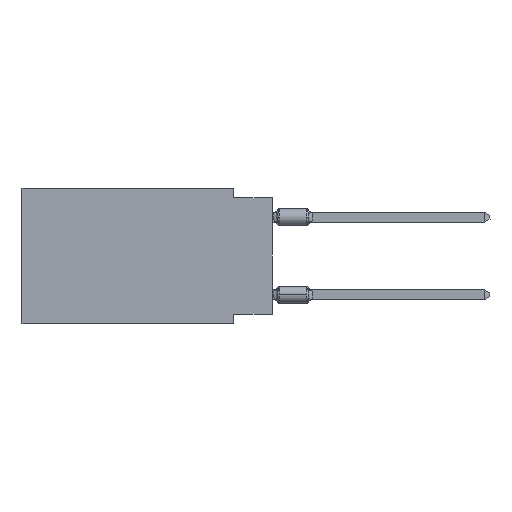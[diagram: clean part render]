
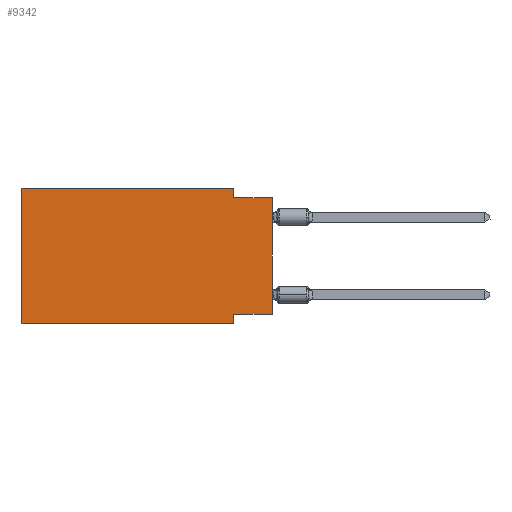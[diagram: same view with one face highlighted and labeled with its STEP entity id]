
A CAD part, left-side view. The second image highlights one B-rep face of the part: STEP entity #9342.
In plain terms, the highlighted planar face has unit normal (-1, 0, 0).
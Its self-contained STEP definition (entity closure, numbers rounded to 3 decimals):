
#448 = CARTESIAN_POINT ( 'NONE',  ( 0., 16.383, -8.89 ) ) ;
#556 = VERTEX_POINT ( 'NONE', #4214 ) ;
#639 = CARTESIAN_POINT ( 'NONE',  ( 0., 16.383, 0. ) ) ;
#869 = VERTEX_POINT ( 'NONE', #639 ) ;
#880 = CARTESIAN_POINT ( 'NONE',  ( 0., 16.383, 0. ) ) ;
#1296 = CARTESIAN_POINT ( 'NONE',  ( 0., 16.383, -8.89 ) ) ;
#2185 = ORIENTED_EDGE ( 'NONE', *, *, #16722, .F. ) ;
#3441 = VECTOR ( 'NONE', #11607, 1000. ) ;
#3609 = VERTEX_POINT ( 'NONE', #29031 ) ;
#3620 = VECTOR ( 'NONE', #23142, 1000. ) ;
#4111 = EDGE_CURVE ( 'NONE', #24552, #21941, #9852, .T. ) ;
#4214 = CARTESIAN_POINT ( 'NONE',  ( 0., 2.54, -8.89 ) ) ;
#4258 = CARTESIAN_POINT ( 'NONE',  ( 0., 0., -0.635 ) ) ;
#4291 = ORIENTED_EDGE ( 'NONE', *, *, #28995, .F. ) ;
#4515 = CARTESIAN_POINT ( 'NONE',  ( 0., 16.383, 0. ) ) ;
#4516 = VERTEX_POINT ( 'NONE', #19698 ) ;
#6310 = DIRECTION ( 'NONE',  ( 0., -1., 0. ) ) ;
#6629 = PLANE ( 'NONE',  #11124 ) ;
#6890 = ORIENTED_EDGE ( 'NONE', *, *, #10405, .F. ) ;
#6940 = DIRECTION ( 'NONE',  ( 0., 0., -1. ) ) ;
#7502 = LINE ( 'NONE', #9932, #27245 ) ;
#7581 = DIRECTION ( 'NONE',  ( 0., 0., 1. ) ) ;
#7999 = DIRECTION ( 'NONE',  ( 0., -1., 0. ) ) ;
#9269 = DIRECTION ( 'NONE',  ( 0., -1., 0. ) ) ;
#9342 = ADVANCED_FACE ( 'NONE', ( #31280 ), #6629, .F. ) ;
#9473 = CARTESIAN_POINT ( 'NONE',  ( 0., 2.54, 0. ) ) ;
#9852 = LINE ( 'NONE', #17305, #14288 ) ;
#9932 = CARTESIAN_POINT ( 'NONE',  ( 0., 2.54, 0. ) ) ;
#10368 = EDGE_CURVE ( 'NONE', #31328, #556, #30657, .T. ) ;
#10405 = EDGE_CURVE ( 'NONE', #31328, #869, #18625, .T. ) ;
#10429 = CARTESIAN_POINT ( 'NONE',  ( 0., 0., -8.255 ) ) ;
#10961 = EDGE_CURVE ( 'NONE', #24552, #3609, #28808, .T. ) ;
#11124 = AXIS2_PLACEMENT_3D ( 'NONE', #4515, #29320, #6940 ) ;
#11432 = CARTESIAN_POINT ( 'NONE',  ( 0., 0., -0.635 ) ) ;
#11607 = DIRECTION ( 'NONE',  ( 0., 1., 0. ) ) ;
#13241 = VECTOR ( 'NONE', #6310, 1000. ) ;
#13596 = CARTESIAN_POINT ( 'NONE',  ( 0., 16.383, 0. ) ) ;
#14288 = VECTOR ( 'NONE', #7581, 1000. ) ;
#15934 = ORIENTED_EDGE ( 'NONE', *, *, #17776, .F. ) ;
#16350 = VECTOR ( 'NONE', #30967, 1000. ) ;
#16722 = EDGE_CURVE ( 'NONE', #3609, #556, #22832, .T. ) ;
#16957 = ORIENTED_EDGE ( 'NONE', *, *, #10961, .F. ) ;
#17305 = CARTESIAN_POINT ( 'NONE',  ( 0., 0., 0. ) ) ;
#17725 = LINE ( 'NONE', #880, #30721 ) ;
#17776 = EDGE_CURVE ( 'NONE', #4516, #21941, #31500, .T. ) ;
#18625 = LINE ( 'NONE', #13596, #16350 ) ;
#18896 = ORIENTED_EDGE ( 'NONE', *, *, #10368, .T. ) ;
#19698 = CARTESIAN_POINT ( 'NONE',  ( 0., 2.54, -0.635 ) ) ;
#19718 = VECTOR ( 'NONE', #9269, 1000. ) ;
#20298 = DIRECTION ( 'NONE',  ( 0., 0., -1. ) ) ;
#20304 = EDGE_CURVE ( 'NONE', #27901, #4516, #7502, .T. ) ;
#21941 = VERTEX_POINT ( 'NONE', #11432 ) ;
#22832 = LINE ( 'NONE', #30750, #3620 ) ;
#23142 = DIRECTION ( 'NONE',  ( 0., 0., -1. ) ) ;
#23155 = EDGE_LOOP ( 'NONE', ( #25103, #15934, #24033, #4291, #6890, #18896, #2185, #16957 ) ) ;
#24033 = ORIENTED_EDGE ( 'NONE', *, *, #20304, .F. ) ;
#24552 = VERTEX_POINT ( 'NONE', #10429 ) ;
#25103 = ORIENTED_EDGE ( 'NONE', *, *, #4111, .T. ) ;
#27245 = VECTOR ( 'NONE', #20298, 1000. ) ;
#27901 = VERTEX_POINT ( 'NONE', #9473 ) ;
#28808 = LINE ( 'NONE', #29126, #3441 ) ;
#28995 = EDGE_CURVE ( 'NONE', #869, #27901, #17725, .T. ) ;
#29031 = CARTESIAN_POINT ( 'NONE',  ( 0., 2.54, -8.255 ) ) ;
#29126 = CARTESIAN_POINT ( 'NONE',  ( 0., 0., -8.255 ) ) ;
#29320 = DIRECTION ( 'NONE',  ( 1., 0., 0. ) ) ;
#30657 = LINE ( 'NONE', #1296, #13241 ) ;
#30721 = VECTOR ( 'NONE', #7999, 1000. ) ;
#30750 = CARTESIAN_POINT ( 'NONE',  ( 0., 2.54, -8.89 ) ) ;
#30967 = DIRECTION ( 'NONE',  ( 0., 0., 1. ) ) ;
#31280 = FACE_OUTER_BOUND ( 'NONE', #23155, .T. ) ;
#31328 = VERTEX_POINT ( 'NONE', #448 ) ;
#31500 = LINE ( 'NONE', #4258, #19718 ) ;
